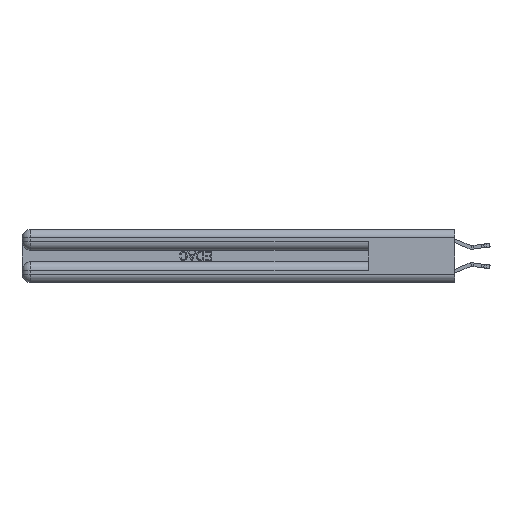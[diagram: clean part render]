
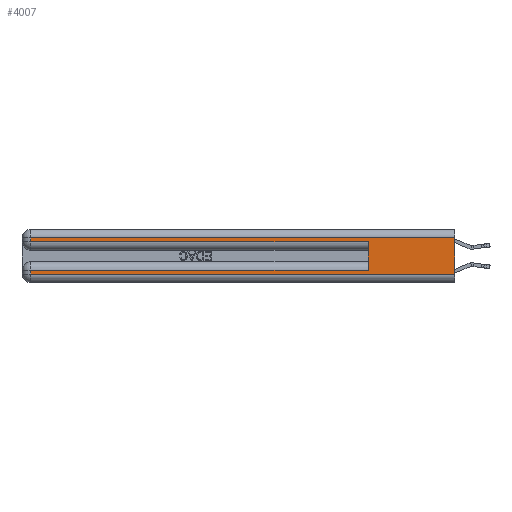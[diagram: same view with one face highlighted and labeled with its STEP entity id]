
A CAD part, left-side view. The second image highlights one B-rep face of the part: STEP entity #4007.
In plain terms, the highlighted planar face has unit normal (-1, 0, 0).
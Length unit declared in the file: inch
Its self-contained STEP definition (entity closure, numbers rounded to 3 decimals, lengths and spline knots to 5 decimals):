
#60 = EDGE_CURVE ( 'NONE', #23070, #23893, #8183, .T. ) ;
#75 = EDGE_CURVE ( 'NONE', #15259, #20160, #8355, .T. ) ;
#481 = EDGE_CURVE ( 'NONE', #14689, #20160, #3227, .T. ) ;
#692 = CARTESIAN_POINT ( 'NONE',  ( 0., 2.94, 0.37 ) ) ;
#1204 = CARTESIAN_POINT ( 'NONE',  ( 0., 0., 0.37 ) ) ;
#1729 = EDGE_CURVE ( 'NONE', #31003, #20545, #28154, .T. ) ;
#1829 = CARTESIAN_POINT ( 'NONE',  ( 0., 2.94, 0.085 ) ) ;
#2966 = DIRECTION ( 'NONE',  ( 0., 0., -1. ) ) ;
#3227 = LINE ( 'NONE', #3403, #17162 ) ;
#3379 = VECTOR ( 'NONE', #29991, 39.37008 ) ;
#3403 = CARTESIAN_POINT ( 'NONE',  ( 0., 0., 0.285 ) ) ;
#4007 = ADVANCED_FACE ( 'NONE', ( #21925 ), #9044, .F. ) ;
#4681 = CARTESIAN_POINT ( 'NONE',  ( 0., 0., 0.31 ) ) ;
#4864 = EDGE_CURVE ( 'NONE', #15259, #23070, #30507, .T. ) ;
#5060 = VECTOR ( 'NONE', #24675, 39.37008 ) ;
#6276 = CARTESIAN_POINT ( 'NONE',  ( 0., 0., 0.06 ) ) ;
#7042 = CARTESIAN_POINT ( 'NONE',  ( 0., 2.94, 0.31 ) ) ;
#7627 = EDGE_LOOP ( 'NONE', ( #33619, #15083, #28882, #14588, #30095, #29254, #15557, #20157 ) ) ;
#8183 = LINE ( 'NONE', #692, #24298 ) ;
#8355 = LINE ( 'NONE', #18987, #14899 ) ;
#8838 = EDGE_CURVE ( 'NONE', #23893, #20545, #9733, .T. ) ;
#9044 = PLANE ( 'NONE',  #26092 ) ;
#9733 = LINE ( 'NONE', #20352, #26284 ) ;
#11287 = CARTESIAN_POINT ( 'NONE',  ( 0., 0., 0.31 ) ) ;
#11316 = DIRECTION ( 'NONE',  ( 1., 0., 0. ) ) ;
#11702 = CARTESIAN_POINT ( 'NONE',  ( 0., 0., 0.085 ) ) ;
#11828 = DIRECTION ( 'NONE',  ( 0., 0., -1. ) ) ;
#11883 = CARTESIAN_POINT ( 'NONE',  ( 0., 0.6, 0.285 ) ) ;
#11995 = DIRECTION ( 'NONE',  ( 0., -1., 0. ) ) ;
#12464 = DIRECTION ( 'NONE',  ( 0., 0., -1. ) ) ;
#14588 = ORIENTED_EDGE ( 'NONE', *, *, #481, .T. ) ;
#14689 = VERTEX_POINT ( 'NONE', #26523 ) ;
#14899 = VECTOR ( 'NONE', #29946, 39.37008 ) ;
#15083 = ORIENTED_EDGE ( 'NONE', *, *, #29210, .T. ) ;
#15259 = VERTEX_POINT ( 'NONE', #29936 ) ;
#15557 = ORIENTED_EDGE ( 'NONE', *, *, #60, .T. ) ;
#16632 = DIRECTION ( 'NONE',  ( 0., -1., 0. ) ) ;
#17162 = VECTOR ( 'NONE', #16632, 39.37008 ) ;
#17562 = VECTOR ( 'NONE', #12464, 39.37008 ) ;
#17870 = CARTESIAN_POINT ( 'NONE',  ( 0., 0., 0.37 ) ) ;
#18594 = VERTEX_POINT ( 'NONE', #7042 ) ;
#18987 = CARTESIAN_POINT ( 'NONE',  ( 0., 0.6, 0.145 ) ) ;
#20157 = ORIENTED_EDGE ( 'NONE', *, *, #8838, .T. ) ;
#20160 = VERTEX_POINT ( 'NONE', #11883 ) ;
#20352 = CARTESIAN_POINT ( 'NONE',  ( 0., 0., 0.06 ) ) ;
#20545 = VERTEX_POINT ( 'NONE', #6276 ) ;
#20714 = CARTESIAN_POINT ( 'NONE',  ( 0., 2.94, 0.06 ) ) ;
#21184 = EDGE_CURVE ( 'NONE', #18594, #14689, #34053, .T. ) ;
#21925 = FACE_OUTER_BOUND ( 'NONE', #7627, .T. ) ;
#23070 = VERTEX_POINT ( 'NONE', #1829 ) ;
#23893 = VERTEX_POINT ( 'NONE', #20714 ) ;
#24298 = VECTOR ( 'NONE', #2966, 39.37008 ) ;
#24675 = DIRECTION ( 'NONE',  ( 0., 1., 0. ) ) ;
#25683 = CARTESIAN_POINT ( 'NONE',  ( 0., 2.94, 0.37 ) ) ;
#26092 = AXIS2_PLACEMENT_3D ( 'NONE', #1204, #11316, #11828 ) ;
#26284 = VECTOR ( 'NONE', #11995, 39.37008 ) ;
#26523 = CARTESIAN_POINT ( 'NONE',  ( 0., 2.94, 0.285 ) ) ;
#26798 = LINE ( 'NONE', #11287, #5060 ) ;
#28061 = VECTOR ( 'NONE', #33882, 39.37008 ) ;
#28154 = LINE ( 'NONE', #17870, #28061 ) ;
#28882 = ORIENTED_EDGE ( 'NONE', *, *, #21184, .T. ) ;
#29210 = EDGE_CURVE ( 'NONE', #31003, #18594, #26798, .T. ) ;
#29254 = ORIENTED_EDGE ( 'NONE', *, *, #4864, .T. ) ;
#29936 = CARTESIAN_POINT ( 'NONE',  ( 0., 0.6, 0.085 ) ) ;
#29946 = DIRECTION ( 'NONE',  ( 0., 0., 1. ) ) ;
#29991 = DIRECTION ( 'NONE',  ( 0., 1., 0. ) ) ;
#30095 = ORIENTED_EDGE ( 'NONE', *, *, #75, .F. ) ;
#30507 = LINE ( 'NONE', #11702, #3379 ) ;
#31003 = VERTEX_POINT ( 'NONE', #4681 ) ;
#33619 = ORIENTED_EDGE ( 'NONE', *, *, #1729, .F. ) ;
#33882 = DIRECTION ( 'NONE',  ( 0., 0., -1. ) ) ;
#34053 = LINE ( 'NONE', #25683, #17562 ) ;
